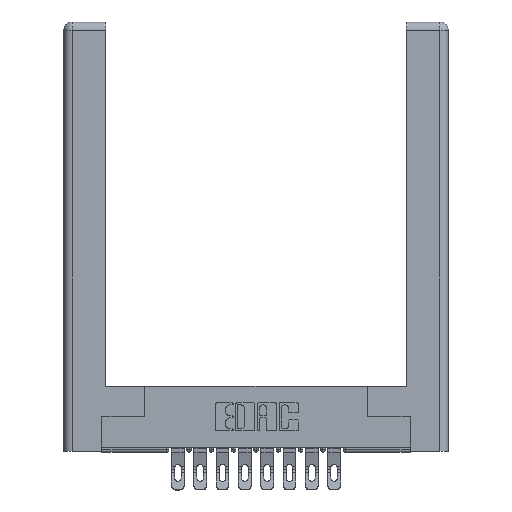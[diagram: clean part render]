
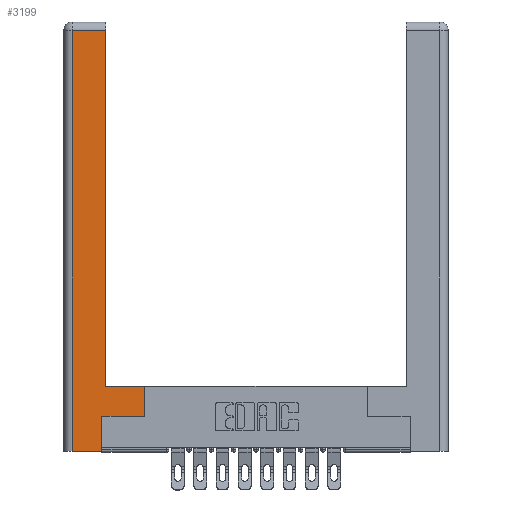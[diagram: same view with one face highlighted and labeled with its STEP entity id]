
A CAD part, top view. The second image highlights one B-rep face of the part: STEP entity #3199.
In plain terms, the highlighted planar face has unit normal (0, 0, 1).
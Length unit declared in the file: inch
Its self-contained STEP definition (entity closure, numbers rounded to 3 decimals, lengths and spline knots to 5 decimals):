
#20 = DIRECTION ( 'NONE',  ( 1., 0., 0. ) ) ;
#678 = EDGE_CURVE ( 'NONE', #15644, #11525, #14762, .T. ) ;
#1184 = VECTOR ( 'NONE', #16017, 39.37008 ) ;
#1409 = EDGE_CURVE ( 'NONE', #7060, #6275, #8791, .T. ) ;
#1438 = EDGE_CURVE ( 'NONE', #6275, #15644, #4686, .T. ) ;
#1737 = VERTEX_POINT ( 'NONE', #15976 ) ;
#2943 = EDGE_CURVE ( 'NONE', #1737, #7060, #13969, .T. ) ;
#3037 = ORIENTED_EDGE ( 'NONE', *, *, #1409, .T. ) ;
#3199 = ADVANCED_FACE ( 'NONE', ( #6183 ), #4528, .F. ) ;
#3876 = EDGE_LOOP ( 'NONE', ( #7275, #11765, #8989, #4133, #11914, #14687, #3037, #6214 ) ) ;
#4133 = ORIENTED_EDGE ( 'NONE', *, *, #10152, .T. ) ;
#4528 = PLANE ( 'NONE',  #8761 ) ;
#4686 = LINE ( 'NONE', #6498, #9584 ) ;
#4859 = VECTOR ( 'NONE', #13751, 39.37008 ) ;
#4943 = CARTESIAN_POINT ( 'NONE',  ( 0.265, 0., 0. ) ) ;
#5620 = CARTESIAN_POINT ( 'NONE',  ( 0.295, 3., 0. ) ) ;
#6183 = FACE_OUTER_BOUND ( 'NONE', #3876, .T. ) ;
#6214 = ORIENTED_EDGE ( 'NONE', *, *, #1438, .T. ) ;
#6250 = VERTEX_POINT ( 'NONE', #4943 ) ;
#6275 = VERTEX_POINT ( 'NONE', #9899 ) ;
#6498 = CARTESIAN_POINT ( 'NONE',  ( 0.295, 0.45, 0. ) ) ;
#6830 = VECTOR ( 'NONE', #14075, 39.37008 ) ;
#7000 = LINE ( 'NONE', #8830, #4859 ) ;
#7060 = VERTEX_POINT ( 'NONE', #9816 ) ;
#7124 = DIRECTION ( 'NONE',  ( 0., 0., -1. ) ) ;
#7275 = ORIENTED_EDGE ( 'NONE', *, *, #678, .T. ) ;
#7475 = EDGE_CURVE ( 'NONE', #11525, #12946, #7868, .T. ) ;
#7868 = LINE ( 'NONE', #12791, #10400 ) ;
#8005 = LINE ( 'NONE', #12392, #1184 ) ;
#8327 = CARTESIAN_POINT ( 'NONE',  ( 0.295, 0.45, 0. ) ) ;
#8761 = AXIS2_PLACEMENT_3D ( 'NONE', #9497, #7124, #10843 ) ;
#8791 = LINE ( 'NONE', #11639, #6830 ) ;
#8830 = CARTESIAN_POINT ( 'NONE',  ( 0.265, 0., 0. ) ) ;
#8989 = ORIENTED_EDGE ( 'NONE', *, *, #12766, .T. ) ;
#9178 = DIRECTION ( 'NONE',  ( 0., 1., 0. ) ) ;
#9284 = VERTEX_POINT ( 'NONE', #12441 ) ;
#9497 = CARTESIAN_POINT ( 'NONE',  ( 0., 0., 0. ) ) ;
#9584 = VECTOR ( 'NONE', #13901, 39.37008 ) ;
#9816 = CARTESIAN_POINT ( 'NONE',  ( 0.565, 0.245, 0. ) ) ;
#9899 = CARTESIAN_POINT ( 'NONE',  ( 0.565, 0.45, 0. ) ) ;
#9964 = CARTESIAN_POINT ( 'NONE',  ( 0.0615, 0., 0. ) ) ;
#10152 = EDGE_CURVE ( 'NONE', #9284, #6250, #7000, .T. ) ;
#10400 = VECTOR ( 'NONE', #14013, 39.37008 ) ;
#10843 = DIRECTION ( 'NONE',  ( -1., 0., 0. ) ) ;
#11460 = CARTESIAN_POINT ( 'NONE',  ( 0.295, 2.94, 0. ) ) ;
#11525 = VERTEX_POINT ( 'NONE', #11460 ) ;
#11639 = CARTESIAN_POINT ( 'NONE',  ( 0.565, 0.45, 0. ) ) ;
#11765 = ORIENTED_EDGE ( 'NONE', *, *, #7475, .T. ) ;
#11914 = ORIENTED_EDGE ( 'NONE', *, *, #15783, .T. ) ;
#12265 = VECTOR ( 'NONE', #9178, 39.37008 ) ;
#12392 = CARTESIAN_POINT ( 'NONE',  ( 0.265, 0.245, 0. ) ) ;
#12441 = CARTESIAN_POINT ( 'NONE',  ( 0.0615, 0., 0. ) ) ;
#12766 = EDGE_CURVE ( 'NONE', #12946, #9284, #16033, .T. ) ;
#12791 = CARTESIAN_POINT ( 'NONE',  ( 0.0615, 2.94, 0. ) ) ;
#12946 = VERTEX_POINT ( 'NONE', #14840 ) ;
#13695 = DIRECTION ( 'NONE',  ( 0., -1., 0. ) ) ;
#13751 = DIRECTION ( 'NONE',  ( 1., 0., 0. ) ) ;
#13763 = VECTOR ( 'NONE', #20, 39.37008 ) ;
#13901 = DIRECTION ( 'NONE',  ( -1., 0., 0. ) ) ;
#13969 = LINE ( 'NONE', #14823, #13763 ) ;
#14013 = DIRECTION ( 'NONE',  ( -1., 0., 0. ) ) ;
#14075 = DIRECTION ( 'NONE',  ( 0., 1., 0. ) ) ;
#14687 = ORIENTED_EDGE ( 'NONE', *, *, #2943, .T. ) ;
#14762 = LINE ( 'NONE', #5620, #12265 ) ;
#14823 = CARTESIAN_POINT ( 'NONE',  ( 0.565, 0.245, 0. ) ) ;
#14840 = CARTESIAN_POINT ( 'NONE',  ( 0.0615, 2.94, 0. ) ) ;
#15256 = VECTOR ( 'NONE', #13695, 39.37008 ) ;
#15644 = VERTEX_POINT ( 'NONE', #8327 ) ;
#15783 = EDGE_CURVE ( 'NONE', #6250, #1737, #8005, .T. ) ;
#15976 = CARTESIAN_POINT ( 'NONE',  ( 0.265, 0.245, 0. ) ) ;
#16017 = DIRECTION ( 'NONE',  ( 0., 1., 0. ) ) ;
#16033 = LINE ( 'NONE', #9964, #15256 ) ;
